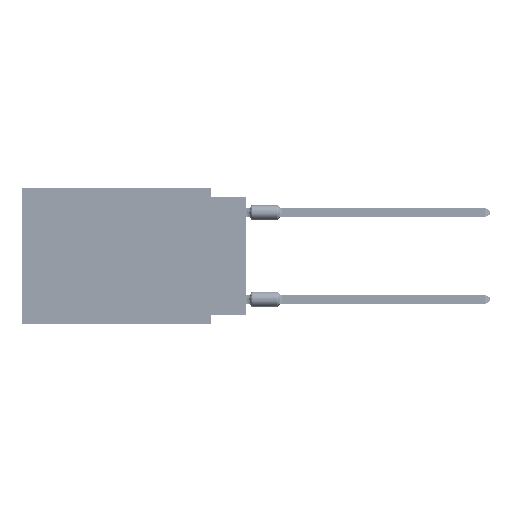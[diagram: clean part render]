
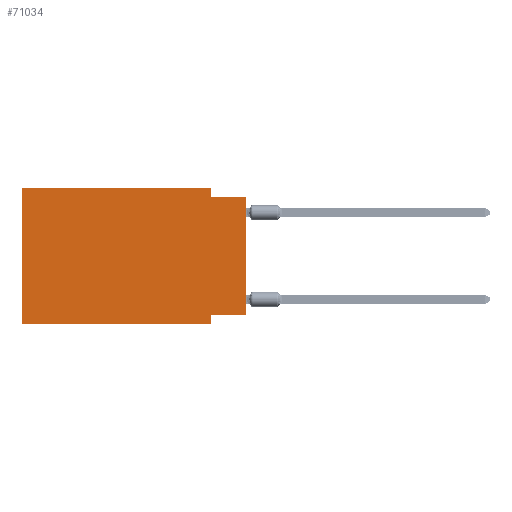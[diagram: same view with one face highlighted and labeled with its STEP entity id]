
A CAD part, left-side view. The second image highlights one B-rep face of the part: STEP entity #71034.
In plain terms, the highlighted planar face has unit normal (-1, 0, 0).
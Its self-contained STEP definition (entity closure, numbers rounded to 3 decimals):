
#488 = VECTOR ( 'NONE', #68139, 1000. ) ;
#2645 = PLANE ( 'NONE',  #79726 ) ;
#3319 = EDGE_CURVE ( 'NONE', #13647, #80582, #24816, .T. ) ;
#4053 = CARTESIAN_POINT ( 'NONE',  ( 0., 16.383, -9.906 ) ) ;
#6256 = VECTOR ( 'NONE', #44791, 1000. ) ;
#7079 = CARTESIAN_POINT ( 'NONE',  ( 0., 16.383, 0. ) ) ;
#7092 = ORIENTED_EDGE ( 'NONE', *, *, #38382, .F. ) ;
#8161 = CARTESIAN_POINT ( 'NONE',  ( 0., 16.383, 0. ) ) ;
#9565 = ORIENTED_EDGE ( 'NONE', *, *, #56065, .T. ) ;
#10509 = CARTESIAN_POINT ( 'NONE',  ( 0., 2.54, 0. ) ) ;
#10590 = ORIENTED_EDGE ( 'NONE', *, *, #3319, .F. ) ;
#13647 = VERTEX_POINT ( 'NONE', #35961 ) ;
#14744 = CARTESIAN_POINT ( 'NONE',  ( 0., 2.54, -0.635 ) ) ;
#16533 = ORIENTED_EDGE ( 'NONE', *, *, #69585, .F. ) ;
#16966 = VERTEX_POINT ( 'NONE', #66463 ) ;
#17300 = CARTESIAN_POINT ( 'NONE',  ( 0., 16.383, 0. ) ) ;
#17404 = CARTESIAN_POINT ( 'NONE',  ( 0., 16.383, 0. ) ) ;
#19173 = LINE ( 'NONE', #8161, #22505 ) ;
#20541 = EDGE_CURVE ( 'NONE', #43269, #54964, #31634, .T. ) ;
#22118 = ORIENTED_EDGE ( 'NONE', *, *, #41603, .T. ) ;
#22505 = VECTOR ( 'NONE', #38336, 1000. ) ;
#24816 = LINE ( 'NONE', #10509, #48464 ) ;
#26417 = VECTOR ( 'NONE', #75755, 1000. ) ;
#27695 = EDGE_CURVE ( 'NONE', #39631, #13647, #19173, .T. ) ;
#27756 = LINE ( 'NONE', #34712, #488 ) ;
#27763 = EDGE_CURVE ( 'NONE', #80582, #16966, #56372, .T. ) ;
#27921 = LINE ( 'NONE', #7079, #66735 ) ;
#29136 = VERTEX_POINT ( 'NONE', #85348 ) ;
#30139 = LINE ( 'NONE', #4053, #26417 ) ;
#31352 = DIRECTION ( 'NONE',  ( 0., 0., -1. ) ) ;
#31634 = LINE ( 'NONE', #72019, #47976 ) ;
#31921 = VERTEX_POINT ( 'NONE', #81642 ) ;
#34712 = CARTESIAN_POINT ( 'NONE',  ( 0., 0., -9.271 ) ) ;
#35961 = CARTESIAN_POINT ( 'NONE',  ( 0., 2.54, 0. ) ) ;
#36410 = CARTESIAN_POINT ( 'NONE',  ( 0., 0., -0.635 ) ) ;
#38336 = DIRECTION ( 'NONE',  ( 0., -1., 0. ) ) ;
#38382 = EDGE_CURVE ( 'NONE', #31921, #39631, #27921, .T. ) ;
#39631 = VERTEX_POINT ( 'NONE', #17300 ) ;
#39700 = DIRECTION ( 'NONE',  ( 0., 0., 1. ) ) ;
#41603 = EDGE_CURVE ( 'NONE', #31921, #54964, #30139, .T. ) ;
#43046 = ORIENTED_EDGE ( 'NONE', *, *, #20541, .F. ) ;
#43066 = DIRECTION ( 'NONE',  ( 1., 0., 0. ) ) ;
#43269 = VERTEX_POINT ( 'NONE', #72152 ) ;
#43949 = DIRECTION ( 'NONE',  ( 0., 0., -1. ) ) ;
#44791 = DIRECTION ( 'NONE',  ( 0., 0., 1. ) ) ;
#45208 = LINE ( 'NONE', #71692, #6256 ) ;
#47976 = VECTOR ( 'NONE', #52907, 1000. ) ;
#48464 = VECTOR ( 'NONE', #31352, 1000. ) ;
#51466 = EDGE_LOOP ( 'NONE', ( #9565, #65785, #10590, #79445, #7092, #22118, #43046, #16533 ) ) ;
#52907 = DIRECTION ( 'NONE',  ( 0., 0., -1. ) ) ;
#54964 = VERTEX_POINT ( 'NONE', #76362 ) ;
#56065 = EDGE_CURVE ( 'NONE', #29136, #16966, #45208, .T. ) ;
#56372 = LINE ( 'NONE', #36410, #62753 ) ;
#62753 = VECTOR ( 'NONE', #75922, 1000. ) ;
#65785 = ORIENTED_EDGE ( 'NONE', *, *, #27763, .F. ) ;
#66463 = CARTESIAN_POINT ( 'NONE',  ( 0., 0., -0.635 ) ) ;
#66735 = VECTOR ( 'NONE', #39700, 1000. ) ;
#68139 = DIRECTION ( 'NONE',  ( 0., 1., 0. ) ) ;
#69585 = EDGE_CURVE ( 'NONE', #29136, #43269, #27756, .T. ) ;
#71034 = ADVANCED_FACE ( 'NONE', ( #75639 ), #2645, .F. ) ;
#71692 = CARTESIAN_POINT ( 'NONE',  ( 0., 0., 0. ) ) ;
#72019 = CARTESIAN_POINT ( 'NONE',  ( 0., 2.54, -9.906 ) ) ;
#72152 = CARTESIAN_POINT ( 'NONE',  ( 0., 2.54, -9.271 ) ) ;
#75639 = FACE_OUTER_BOUND ( 'NONE', #51466, .T. ) ;
#75755 = DIRECTION ( 'NONE',  ( 0., -1., 0. ) ) ;
#75922 = DIRECTION ( 'NONE',  ( 0., -1., 0. ) ) ;
#76362 = CARTESIAN_POINT ( 'NONE',  ( 0., 2.54, -9.906 ) ) ;
#79445 = ORIENTED_EDGE ( 'NONE', *, *, #27695, .F. ) ;
#79726 = AXIS2_PLACEMENT_3D ( 'NONE', #17404, #43066, #43949 ) ;
#80582 = VERTEX_POINT ( 'NONE', #14744 ) ;
#81642 = CARTESIAN_POINT ( 'NONE',  ( 0., 16.383, -9.906 ) ) ;
#85348 = CARTESIAN_POINT ( 'NONE',  ( 0., 0., -9.271 ) ) ;
